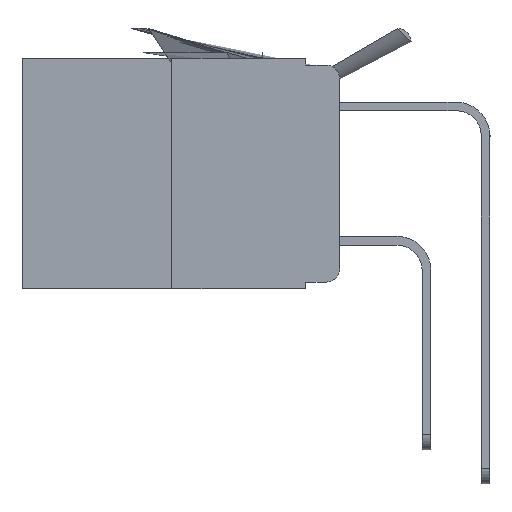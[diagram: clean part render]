
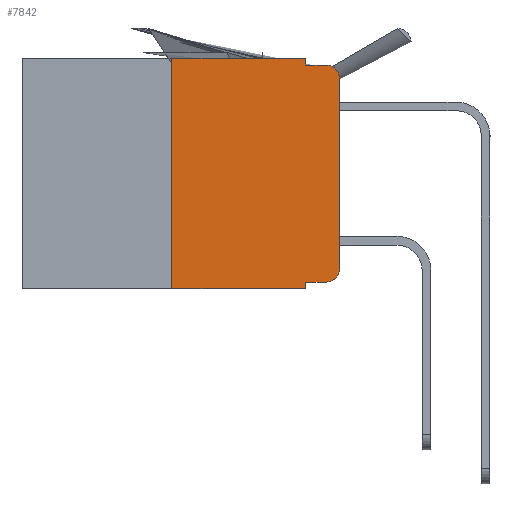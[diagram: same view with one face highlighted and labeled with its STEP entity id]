
A CAD part, left-side view. The second image highlights one B-rep face of the part: STEP entity #7842.
In plain terms, the highlighted planar face has unit normal (-1, 0, 0).
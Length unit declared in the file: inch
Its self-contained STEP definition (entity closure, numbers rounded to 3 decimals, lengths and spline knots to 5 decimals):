
#228 = VERTEX_POINT ( 'NONE', #5017 ) ;
#585 = VERTEX_POINT ( 'NONE', #12131 ) ;
#976 = ORIENTED_EDGE ( 'NONE', *, *, #15684, .F. ) ;
#977 = AXIS2_PLACEMENT_3D ( 'NONE', #9350, #9627, #9655 ) ;
#1192 = ORIENTED_EDGE ( 'NONE', *, *, #17592, .F. ) ;
#1505 = DIRECTION ( 'NONE',  ( 0., -1., 0. ) ) ;
#1590 = DIRECTION ( 'NONE',  ( 0., 0., 1. ) ) ;
#2201 = ORIENTED_EDGE ( 'NONE', *, *, #12707, .T. ) ;
#2542 = CARTESIAN_POINT ( 'NONE',  ( 0., 0.25, 0. ) ) ;
#2769 = ORIENTED_EDGE ( 'NONE', *, *, #5443, .F. ) ;
#2813 = VERTEX_POINT ( 'NONE', #18645 ) ;
#2960 = VECTOR ( 'NONE', #1505, 39.37008 ) ;
#4112 = EDGE_CURVE ( 'NONE', #12652, #18027, #15049, .T. ) ;
#4194 = CARTESIAN_POINT ( 'NONE',  ( 0., 0.051, 0. ) ) ;
#4484 = VECTOR ( 'NONE', #10304, 39.37008 ) ;
#4845 = ORIENTED_EDGE ( 'NONE', *, *, #13702, .T. ) ;
#5017 = CARTESIAN_POINT ( 'NONE',  ( 0., 0.051, -0.333 ) ) ;
#5081 = CARTESIAN_POINT ( 'NONE',  ( 0., 0., 0. ) ) ;
#5375 = CARTESIAN_POINT ( 'NONE',  ( 0., 0.051, -0.01 ) ) ;
#5443 = EDGE_CURVE ( 'NONE', #10859, #585, #12629, .T. ) ;
#5528 = DIRECTION ( 'NONE',  ( 0., -1., 0. ) ) ;
#5730 = ORIENTED_EDGE ( 'NONE', *, *, #8289, .F. ) ;
#6282 = CIRCLE ( 'NONE', #19975, 0.02 ) ;
#6308 = CARTESIAN_POINT ( 'NONE',  ( 0., 0., -0.03 ) ) ;
#6324 = CARTESIAN_POINT ( 'NONE',  ( 0., 0.051, 0. ) ) ;
#6548 = VECTOR ( 'NONE', #1590, 39.37008 ) ;
#6655 = VECTOR ( 'NONE', #7910, 39.37008 ) ;
#6736 = VECTOR ( 'NONE', #10489, 39.37008 ) ;
#7235 = LINE ( 'NONE', #4194, #6736 ) ;
#7520 = ORIENTED_EDGE ( 'NONE', *, *, #8901, .T. ) ;
#7547 = VECTOR ( 'NONE', #7621, 39.37008 ) ;
#7621 = DIRECTION ( 'NONE',  ( 0., 0., 1. ) ) ;
#7826 = ORIENTED_EDGE ( 'NONE', *, *, #15290, .F. ) ;
#7842 = ADVANCED_FACE ( 'NONE', ( #9742 ), #13886, .F. ) ;
#7910 = DIRECTION ( 'NONE',  ( 0., 0., -1. ) ) ;
#8289 = EDGE_CURVE ( 'NONE', #19432, #10859, #11599, .T. ) ;
#8672 = LINE ( 'NONE', #10176, #19890 ) ;
#8889 = CARTESIAN_POINT ( 'NONE',  ( 0., 0.02, -0.03 ) ) ;
#8901 = EDGE_CURVE ( 'NONE', #19432, #2813, #18177, .T. ) ;
#9350 = CARTESIAN_POINT ( 'NONE',  ( 0., 0.02, -0.313 ) ) ;
#9456 = VECTOR ( 'NONE', #10984, 39.37008 ) ;
#9474 = DIRECTION ( 'NONE',  ( 1., 0., 0. ) ) ;
#9627 = DIRECTION ( 'NONE',  ( -1., 0., 0. ) ) ;
#9655 = DIRECTION ( 'NONE',  ( 0., 0., -1. ) ) ;
#9742 = FACE_OUTER_BOUND ( 'NONE', #10069, .T. ) ;
#10069 = EDGE_LOOP ( 'NONE', ( #2201, #4845, #976, #1192, #2769, #5730, #7520, #7826, #10251, #10265 ) ) ;
#10176 = CARTESIAN_POINT ( 'NONE',  ( 0., 0.051, -0.01 ) ) ;
#10251 = ORIENTED_EDGE ( 'NONE', *, *, #10364, .T. ) ;
#10265 = ORIENTED_EDGE ( 'NONE', *, *, #4112, .T. ) ;
#10304 = DIRECTION ( 'NONE',  ( 0., -1., 0. ) ) ;
#10364 = EDGE_CURVE ( 'NONE', #228, #12652, #19463, .T. ) ;
#10419 = DIRECTION ( 'NONE',  ( 0., 0., -1. ) ) ;
#10489 = DIRECTION ( 'NONE',  ( 0., 0., -1. ) ) ;
#10551 = VERTEX_POINT ( 'NONE', #20092 ) ;
#10742 = LINE ( 'NONE', #6324, #6655 ) ;
#10859 = VERTEX_POINT ( 'NONE', #2542 ) ;
#10984 = DIRECTION ( 'NONE',  ( 0., -1., 0. ) ) ;
#11081 = CARTESIAN_POINT ( 'NONE',  ( 0., 0.051, -0.333 ) ) ;
#11599 = LINE ( 'NONE', #17997, #7547 ) ;
#12131 = CARTESIAN_POINT ( 'NONE',  ( 0., 0.051, 0. ) ) ;
#12629 = LINE ( 'NONE', #15587, #4484 ) ;
#12652 = VERTEX_POINT ( 'NONE', #19791 ) ;
#12707 = EDGE_CURVE ( 'NONE', #18027, #14859, #14119, .T. ) ;
#12908 = AXIS2_PLACEMENT_3D ( 'NONE', #18254, #9474, #19676 ) ;
#13702 = EDGE_CURVE ( 'NONE', #14859, #10551, #6282, .T. ) ;
#13886 = PLANE ( 'NONE',  #12908 ) ;
#14119 = LINE ( 'NONE', #5081, #6548 ) ;
#14380 = VERTEX_POINT ( 'NONE', #5375 ) ;
#14859 = VERTEX_POINT ( 'NONE', #6308 ) ;
#15049 = CIRCLE ( 'NONE', #977, 0.02 ) ;
#15290 = EDGE_CURVE ( 'NONE', #228, #2813, #7235, .T. ) ;
#15587 = CARTESIAN_POINT ( 'NONE',  ( 0., 0.473, 0. ) ) ;
#15684 = EDGE_CURVE ( 'NONE', #14380, #10551, #8672, .T. ) ;
#16673 = CARTESIAN_POINT ( 'NONE',  ( 0., 0.25, -0.343 ) ) ;
#17592 = EDGE_CURVE ( 'NONE', #585, #14380, #10742, .T. ) ;
#17624 = CARTESIAN_POINT ( 'NONE',  ( 0., 0., -0.313 ) ) ;
#17997 = CARTESIAN_POINT ( 'NONE',  ( 0., 0.25, 0. ) ) ;
#18027 = VERTEX_POINT ( 'NONE', #17624 ) ;
#18177 = LINE ( 'NONE', #18268, #9456 ) ;
#18254 = CARTESIAN_POINT ( 'NONE',  ( 0., 0.473, 0. ) ) ;
#18268 = CARTESIAN_POINT ( 'NONE',  ( 0., 0.473, -0.343 ) ) ;
#18645 = CARTESIAN_POINT ( 'NONE',  ( 0., 0.051, -0.343 ) ) ;
#19145 = DIRECTION ( 'NONE',  ( -1., 0., 0. ) ) ;
#19432 = VERTEX_POINT ( 'NONE', #16673 ) ;
#19463 = LINE ( 'NONE', #11081, #2960 ) ;
#19676 = DIRECTION ( 'NONE',  ( 0., 0., -1. ) ) ;
#19791 = CARTESIAN_POINT ( 'NONE',  ( 0., 0.02, -0.333 ) ) ;
#19890 = VECTOR ( 'NONE', #5528, 39.37008 ) ;
#19975 = AXIS2_PLACEMENT_3D ( 'NONE', #8889, #19145, #10419 ) ;
#20092 = CARTESIAN_POINT ( 'NONE',  ( 0., 0.02, -0.01 ) ) ;
